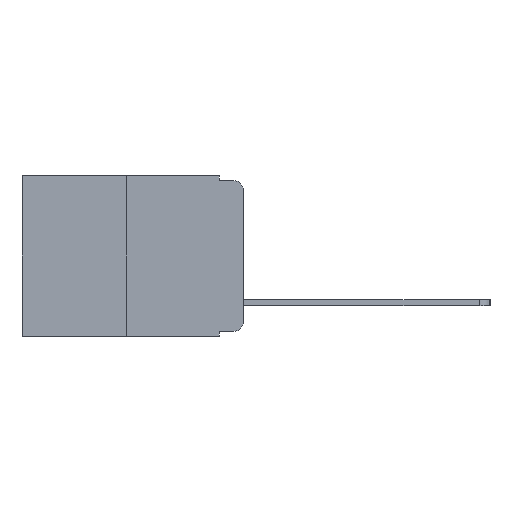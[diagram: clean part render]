
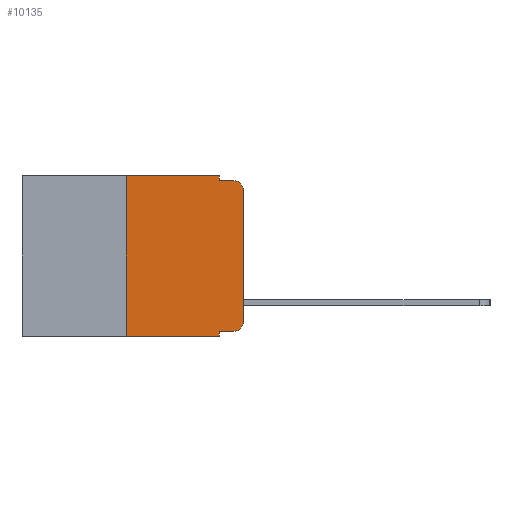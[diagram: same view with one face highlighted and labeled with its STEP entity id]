
A CAD part, left-side view. The second image highlights one B-rep face of the part: STEP entity #10135.
In plain terms, the highlighted planar face has unit normal (-1, 0, 0).
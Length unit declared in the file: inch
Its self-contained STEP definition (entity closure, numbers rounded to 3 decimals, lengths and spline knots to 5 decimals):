
#148 = CIRCLE ( 'NONE', #6169, 0.02 ) ;
#380 = CARTESIAN_POINT ( 'NONE',  ( 0., 0., -0.313 ) ) ;
#414 = EDGE_CURVE ( 'NONE', #6457, #5185, #10348, .T. ) ;
#490 = DIRECTION ( 'NONE',  ( 0., 0., -1. ) ) ;
#534 = ORIENTED_EDGE ( 'NONE', *, *, #11621, .T. ) ;
#811 = DIRECTION ( 'NONE',  ( 1., 0., 0. ) ) ;
#817 = LINE ( 'NONE', #1328, #10479 ) ;
#1145 = VERTEX_POINT ( 'NONE', #5321 ) ;
#1212 = CARTESIAN_POINT ( 'NONE',  ( 0., 0.051, 0. ) ) ;
#1328 = CARTESIAN_POINT ( 'NONE',  ( 0., 0.473, -0.343 ) ) ;
#1820 = EDGE_CURVE ( 'NONE', #1145, #10410, #5720, .T. ) ;
#2080 = EDGE_LOOP ( 'NONE', ( #2935, #2796, #2296, #2161, #2090, #8108, #534, #4888, #4741, #4347 ) ) ;
#2090 = ORIENTED_EDGE ( 'NONE', *, *, #8020, .F. ) ;
#2158 = CARTESIAN_POINT ( 'NONE',  ( 0., 0.25, -0.343 ) ) ;
#2161 = ORIENTED_EDGE ( 'NONE', *, *, #8591, .F. ) ;
#2296 = ORIENTED_EDGE ( 'NONE', *, *, #10455, .F. ) ;
#2570 = DIRECTION ( 'NONE',  ( 0., -1., 0. ) ) ;
#2796 = ORIENTED_EDGE ( 'NONE', *, *, #1820, .T. ) ;
#2863 = CARTESIAN_POINT ( 'NONE',  ( 0., 0.051, -0.333 ) ) ;
#2935 = ORIENTED_EDGE ( 'NONE', *, *, #11576, .T. ) ;
#3024 = CARTESIAN_POINT ( 'NONE',  ( 0., 0.02, -0.313 ) ) ;
#3096 = DIRECTION ( 'NONE',  ( 0., 0., -1. ) ) ;
#3103 = DIRECTION ( 'NONE',  ( -1., 0., 0. ) ) ;
#3211 = VERTEX_POINT ( 'NONE', #2863 ) ;
#3505 = VECTOR ( 'NONE', #490, 39.37008 ) ;
#3879 = LINE ( 'NONE', #4267, #11021 ) ;
#3902 = CARTESIAN_POINT ( 'NONE',  ( 0., 0.051, -0.01 ) ) ;
#4012 = VERTEX_POINT ( 'NONE', #380 ) ;
#4023 = LINE ( 'NONE', #8444, #10632 ) ;
#4047 = VERTEX_POINT ( 'NONE', #1212 ) ;
#4089 = CARTESIAN_POINT ( 'NONE',  ( 0., 0.473, 0. ) ) ;
#4091 = CARTESIAN_POINT ( 'NONE',  ( 0., 0.25, 0. ) ) ;
#4128 = LINE ( 'NONE', #6335, #10211 ) ;
#4267 = CARTESIAN_POINT ( 'NONE',  ( 0., 0.051, 0. ) ) ;
#4347 = ORIENTED_EDGE ( 'NONE', *, *, #5329, .T. ) ;
#4471 = LINE ( 'NONE', #4089, #11031 ) ;
#4741 = ORIENTED_EDGE ( 'NONE', *, *, #8789, .T. ) ;
#4888 = ORIENTED_EDGE ( 'NONE', *, *, #10437, .F. ) ;
#5137 = VERTEX_POINT ( 'NONE', #3902 ) ;
#5185 = VERTEX_POINT ( 'NONE', #5613 ) ;
#5321 = CARTESIAN_POINT ( 'NONE',  ( 0., 0., -0.03 ) ) ;
#5329 = EDGE_CURVE ( 'NONE', #7934, #4012, #148, .T. ) ;
#5390 = DIRECTION ( 'NONE',  ( 0., 0., -1. ) ) ;
#5426 = CARTESIAN_POINT ( 'NONE',  ( 0., 0.051, 0. ) ) ;
#5613 = CARTESIAN_POINT ( 'NONE',  ( 0., 0.25, 0. ) ) ;
#5720 = CIRCLE ( 'NONE', #8247, 0.02 ) ;
#6033 = FACE_OUTER_BOUND ( 'NONE', #2080, .T. ) ;
#6169 = AXIS2_PLACEMENT_3D ( 'NONE', #3024, #3103, #3096 ) ;
#6181 = VERTEX_POINT ( 'NONE', #8620 ) ;
#6335 = CARTESIAN_POINT ( 'NONE',  ( 0., 0.051, -0.01 ) ) ;
#6457 = VERTEX_POINT ( 'NONE', #2158 ) ;
#6610 = CARTESIAN_POINT ( 'NONE',  ( 0., 0.473, 0. ) ) ;
#7119 = LINE ( 'NONE', #9349, #8807 ) ;
#7480 = DIRECTION ( 'NONE',  ( 0., 0., -1. ) ) ;
#7484 = DIRECTION ( 'NONE',  ( 0., 0., -1. ) ) ;
#7883 = DIRECTION ( 'NONE',  ( 0., -1., 0. ) ) ;
#7934 = VERTEX_POINT ( 'NONE', #9324 ) ;
#8020 = EDGE_CURVE ( 'NONE', #5185, #4047, #4471, .T. ) ;
#8108 = ORIENTED_EDGE ( 'NONE', *, *, #414, .F. ) ;
#8198 = VECTOR ( 'NONE', #11256, 39.37008 ) ;
#8247 = AXIS2_PLACEMENT_3D ( 'NONE', #10401, #10383, #5390 ) ;
#8444 = CARTESIAN_POINT ( 'NONE',  ( 0., 0.051, -0.333 ) ) ;
#8468 = DIRECTION ( 'NONE',  ( 0., -1., 0. ) ) ;
#8591 = EDGE_CURVE ( 'NONE', #4047, #5137, #3879, .T. ) ;
#8620 = CARTESIAN_POINT ( 'NONE',  ( 0., 0.051, -0.343 ) ) ;
#8789 = EDGE_CURVE ( 'NONE', #3211, #7934, #4023, .T. ) ;
#8807 = VECTOR ( 'NONE', #9379, 39.37008 ) ;
#9222 = AXIS2_PLACEMENT_3D ( 'NONE', #6610, #811, #7480 ) ;
#9324 = CARTESIAN_POINT ( 'NONE',  ( 0., 0.02, -0.333 ) ) ;
#9340 = DIRECTION ( 'NONE',  ( 0., -1., 0. ) ) ;
#9349 = CARTESIAN_POINT ( 'NONE',  ( 0., 0., 0. ) ) ;
#9379 = DIRECTION ( 'NONE',  ( 0., 0., 1. ) ) ;
#10135 = ADVANCED_FACE ( 'NONE', ( #6033 ), #11593, .F. ) ;
#10211 = VECTOR ( 'NONE', #2570, 39.37008 ) ;
#10348 = LINE ( 'NONE', #4091, #8198 ) ;
#10383 = DIRECTION ( 'NONE',  ( -1., 0., 0. ) ) ;
#10401 = CARTESIAN_POINT ( 'NONE',  ( 0., 0.02, -0.03 ) ) ;
#10410 = VERTEX_POINT ( 'NONE', #11291 ) ;
#10437 = EDGE_CURVE ( 'NONE', #3211, #6181, #10725, .T. ) ;
#10455 = EDGE_CURVE ( 'NONE', #5137, #10410, #4128, .T. ) ;
#10479 = VECTOR ( 'NONE', #7883, 39.37008 ) ;
#10632 = VECTOR ( 'NONE', #8468, 39.37008 ) ;
#10725 = LINE ( 'NONE', #5426, #3505 ) ;
#11021 = VECTOR ( 'NONE', #7484, 39.37008 ) ;
#11031 = VECTOR ( 'NONE', #9340, 39.37008 ) ;
#11256 = DIRECTION ( 'NONE',  ( 0., 0., 1. ) ) ;
#11291 = CARTESIAN_POINT ( 'NONE',  ( 0., 0.02, -0.01 ) ) ;
#11576 = EDGE_CURVE ( 'NONE', #4012, #1145, #7119, .T. ) ;
#11593 = PLANE ( 'NONE',  #9222 ) ;
#11621 = EDGE_CURVE ( 'NONE', #6457, #6181, #817, .T. ) ;
